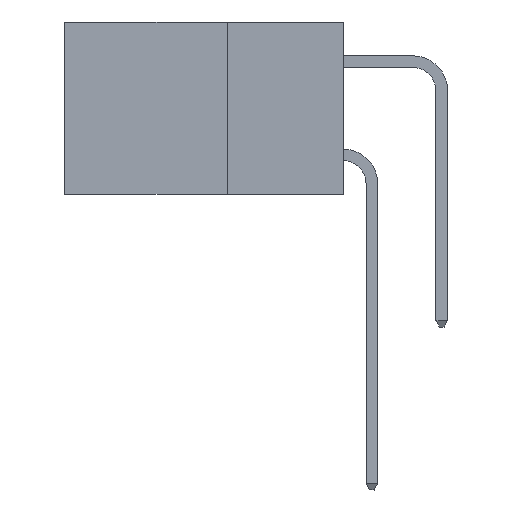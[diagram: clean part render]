
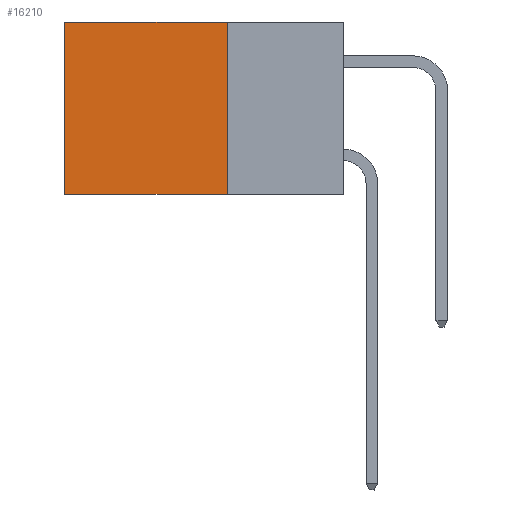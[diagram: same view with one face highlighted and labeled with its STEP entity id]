
A CAD part, left-side view. The second image highlights one B-rep face of the part: STEP entity #16210.
In plain terms, the highlighted planar face has unit normal (-1, 0, 0).
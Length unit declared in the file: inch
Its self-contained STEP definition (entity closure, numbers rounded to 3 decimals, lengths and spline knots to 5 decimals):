
#384 = FACE_OUTER_BOUND ( 'NONE', #12632, .T. ) ;
#1983 = CARTESIAN_POINT ( 'NONE',  ( 0.298, 0.25, 0. ) ) ;
#3073 = ORIENTED_EDGE ( 'NONE', *, *, #11284, .F. ) ;
#3449 = LINE ( 'NONE', #10613, #10276 ) ;
#3469 = DIRECTION ( 'NONE',  ( 0., 0., -1. ) ) ;
#3785 = VECTOR ( 'NONE', #7360, 39.37008 ) ;
#4080 = CARTESIAN_POINT ( 'NONE',  ( 0.298, 0.25, 0. ) ) ;
#4324 = CARTESIAN_POINT ( 'NONE',  ( 0.298, 0.25, -0.37 ) ) ;
#4460 = ORIENTED_EDGE ( 'NONE', *, *, #10235, .T. ) ;
#4546 = CARTESIAN_POINT ( 'NONE',  ( 0.298, 0.6, 0. ) ) ;
#5114 = CARTESIAN_POINT ( 'NONE',  ( 0.298, 0.6, -0.37 ) ) ;
#6478 = VECTOR ( 'NONE', #11517, 39.37008 ) ;
#6965 = ORIENTED_EDGE ( 'NONE', *, *, #8363, .F. ) ;
#7008 = AXIS2_PLACEMENT_3D ( 'NONE', #16894, #7395, #3469 ) ;
#7360 = DIRECTION ( 'NONE',  ( 0., 0., -1. ) ) ;
#7395 = DIRECTION ( 'NONE',  ( 1., 0., 0. ) ) ;
#8363 = EDGE_CURVE ( 'NONE', #13036, #12088, #3449, .T. ) ;
#9514 = LINE ( 'NONE', #1983, #6478 ) ;
#10235 = EDGE_CURVE ( 'NONE', #14768, #12088, #10421, .T. ) ;
#10243 = ORIENTED_EDGE ( 'NONE', *, *, #16530, .T. ) ;
#10276 = VECTOR ( 'NONE', #11435, 39.37008 ) ;
#10421 = LINE ( 'NONE', #16331, #3785 ) ;
#10613 = CARTESIAN_POINT ( 'NONE',  ( 0.298, 0.25, -0.37 ) ) ;
#11284 = EDGE_CURVE ( 'NONE', #11425, #13036, #9514, .T. ) ;
#11425 = VERTEX_POINT ( 'NONE', #16427 ) ;
#11435 = DIRECTION ( 'NONE',  ( 0., 1., 0. ) ) ;
#11517 = DIRECTION ( 'NONE',  ( 0., 0., -1. ) ) ;
#11662 = VECTOR ( 'NONE', #14998, 39.37008 ) ;
#12088 = VERTEX_POINT ( 'NONE', #5114 ) ;
#12632 = EDGE_LOOP ( 'NONE', ( #4460, #6965, #3073, #10243 ) ) ;
#13036 = VERTEX_POINT ( 'NONE', #4324 ) ;
#14203 = LINE ( 'NONE', #4080, #11662 ) ;
#14768 = VERTEX_POINT ( 'NONE', #4546 ) ;
#14998 = DIRECTION ( 'NONE',  ( 0., 1., 0. ) ) ;
#16210 = ADVANCED_FACE ( 'NONE', ( #384 ), #17013, .F. ) ;
#16331 = CARTESIAN_POINT ( 'NONE',  ( 0.298, 0.6, 0. ) ) ;
#16427 = CARTESIAN_POINT ( 'NONE',  ( 0.298, 0.25, 0. ) ) ;
#16530 = EDGE_CURVE ( 'NONE', #11425, #14768, #14203, .T. ) ;
#16894 = CARTESIAN_POINT ( 'NONE',  ( 0.298, 0.25, 0. ) ) ;
#17013 = PLANE ( 'NONE',  #7008 ) ;
